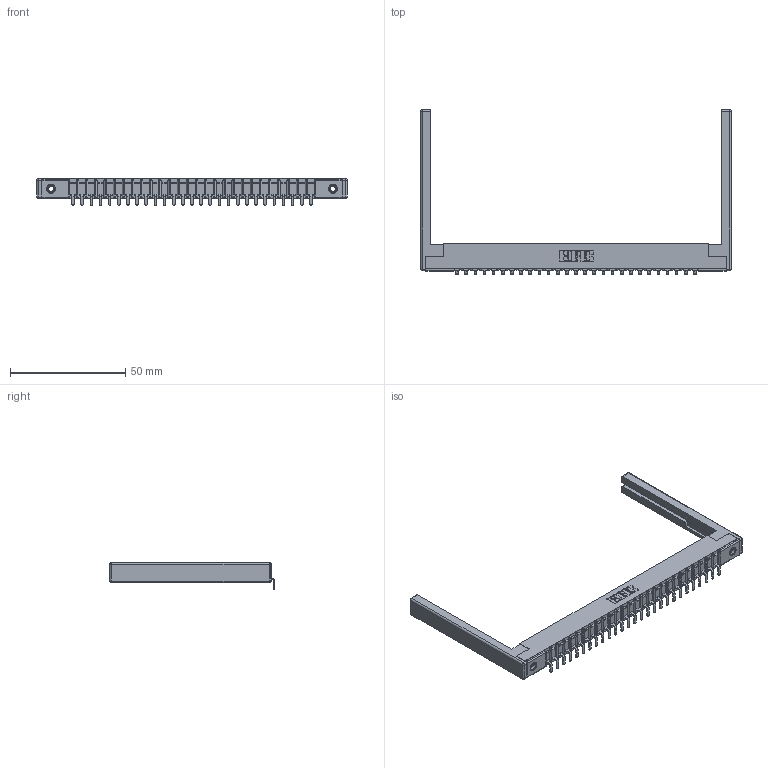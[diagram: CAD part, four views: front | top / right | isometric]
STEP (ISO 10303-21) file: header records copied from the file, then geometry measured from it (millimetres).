
FILE_DESCRIPTION (( 'STEP AP203' ), '1' );
FILE_NAME ('357-027-553-168.STEP', '2019-09-17T01:44:24', ( '' ), ( '' ), 'SwSTEP 2.0', 'SolidWorks 2016', '' );
FILE_SCHEMA (( 'CONFIG_CONTROL_DESIGN' ));
Length unit declared in the file: inch
Products named in the file (5): 357-027-553-168; 307-220-068; 307 Part_.156 Dia Mounting Holes; 307-290-002_553; 345-250-001_345-250-001-102
Assembly tree (32 placements, depth 2):
  357-027-553-168
    307 Part_.156 Dia Mounting Holes
    307-290-002_553  x27
    307-220-068  x2
    345-250-001_345-250-001-102  x2
Bounding box: 134.42 x 71.29 x 11.51 mm (x, y, z)
Volume: 13435.2 mm3; surface area: 20451.5 mm2
Topology: 32 solids, 32 shells, 2406 faces, 7301 edges, 4770 vertices
Faces by surface type: plane 1427, cylinder 899, sphere 64, cone 12, torus 4
Entity records: 28609 total; most frequent: CARTESIAN_POINT 4789, ORIENTED_EDGE 4768, DIRECTION 4678, EDGE_CURVE 2384, VECTOR 1816, LINE 1816, VERTEX_POINT 1542, AXIS2_PLACEMENT_3D 1431
